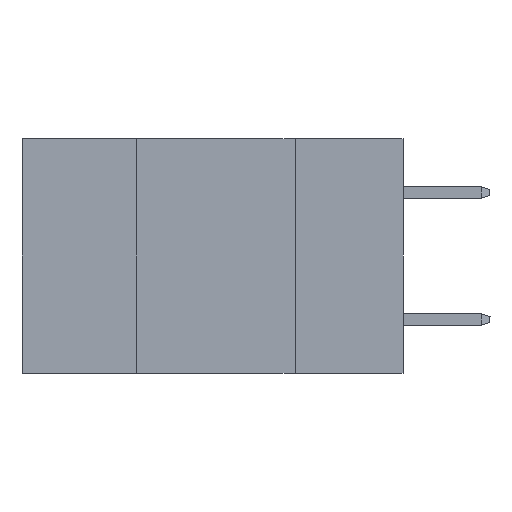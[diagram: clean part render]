
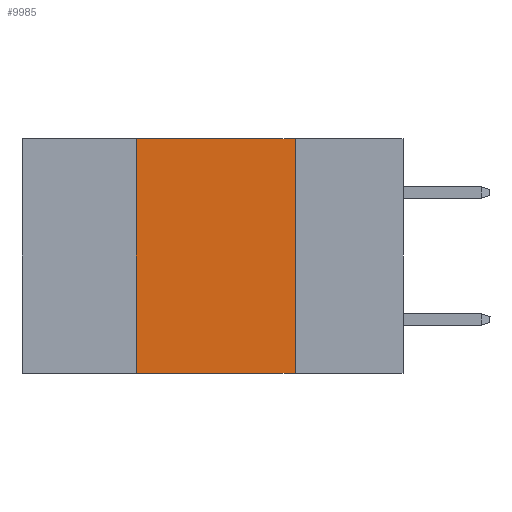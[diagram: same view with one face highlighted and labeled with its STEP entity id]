
A CAD part, left-side view. The second image highlights one B-rep face of the part: STEP entity #9985.
In plain terms, the highlighted planar face has unit normal (-1, 0, 0).
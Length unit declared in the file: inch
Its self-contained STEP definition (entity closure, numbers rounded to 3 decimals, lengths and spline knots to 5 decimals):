
#315 = LINE ( 'NONE', #4958, #4850 ) ;
#464 = VERTEX_POINT ( 'NONE', #3043 ) ;
#575 = EDGE_LOOP ( 'NONE', ( #10198, #1272, #4647, #2709 ) ) ;
#1272 = ORIENTED_EDGE ( 'NONE', *, *, #13683, .F. ) ;
#2347 = LINE ( 'NONE', #6946, #7502 ) ;
#2424 = VERTEX_POINT ( 'NONE', #3174 ) ;
#2430 = VERTEX_POINT ( 'NONE', #11182 ) ;
#2709 = ORIENTED_EDGE ( 'NONE', *, *, #9963, .T. ) ;
#2966 = FACE_OUTER_BOUND ( 'NONE', #575, .T. ) ;
#3043 = CARTESIAN_POINT ( 'NONE',  ( 0., 0.17, 0. ) ) ;
#3174 = CARTESIAN_POINT ( 'NONE',  ( 0., 0.17, -0.37 ) ) ;
#4108 = VERTEX_POINT ( 'NONE', #7372 ) ;
#4647 = ORIENTED_EDGE ( 'NONE', *, *, #7159, .F. ) ;
#4850 = VECTOR ( 'NONE', #12936, 39.37008 ) ;
#4958 = CARTESIAN_POINT ( 'NONE',  ( 0., 0.6, 0. ) ) ;
#5281 = PLANE ( 'NONE',  #6709 ) ;
#5360 = LINE ( 'NONE', #14566, #7930 ) ;
#5420 = LINE ( 'NONE', #12174, #12059 ) ;
#6709 = AXIS2_PLACEMENT_3D ( 'NONE', #13168, #7635, #11212 ) ;
#6946 = CARTESIAN_POINT ( 'NONE',  ( 0., 0.17, 0. ) ) ;
#7159 = EDGE_CURVE ( 'NONE', #2430, #4108, #5420, .T. ) ;
#7372 = CARTESIAN_POINT ( 'NONE',  ( 0., 0.42, 0. ) ) ;
#7502 = VECTOR ( 'NONE', #11564, 39.37008 ) ;
#7635 = DIRECTION ( 'NONE',  ( 1., 0., 0. ) ) ;
#7713 = DIRECTION ( 'NONE',  ( 0., -1., 0. ) ) ;
#7930 = VECTOR ( 'NONE', #7713, 39.37008 ) ;
#9963 = EDGE_CURVE ( 'NONE', #2430, #2424, #5360, .T. ) ;
#9985 = ADVANCED_FACE ( 'NONE', ( #2966 ), #5281, .F. ) ;
#10198 = ORIENTED_EDGE ( 'NONE', *, *, #14029, .F. ) ;
#11182 = CARTESIAN_POINT ( 'NONE',  ( 0., 0.42, -0.37 ) ) ;
#11212 = DIRECTION ( 'NONE',  ( 0., 0., -1. ) ) ;
#11564 = DIRECTION ( 'NONE',  ( 0., 0., -1. ) ) ;
#12059 = VECTOR ( 'NONE', #13457, 39.37008 ) ;
#12174 = CARTESIAN_POINT ( 'NONE',  ( 0., 0.42, 0. ) ) ;
#12936 = DIRECTION ( 'NONE',  ( 0., -1., 0. ) ) ;
#13168 = CARTESIAN_POINT ( 'NONE',  ( 0., 0.6, 0. ) ) ;
#13457 = DIRECTION ( 'NONE',  ( 0., 0., 1. ) ) ;
#13683 = EDGE_CURVE ( 'NONE', #4108, #464, #315, .T. ) ;
#14029 = EDGE_CURVE ( 'NONE', #464, #2424, #2347, .T. ) ;
#14566 = CARTESIAN_POINT ( 'NONE',  ( 0., 0.6, -0.37 ) ) ;
